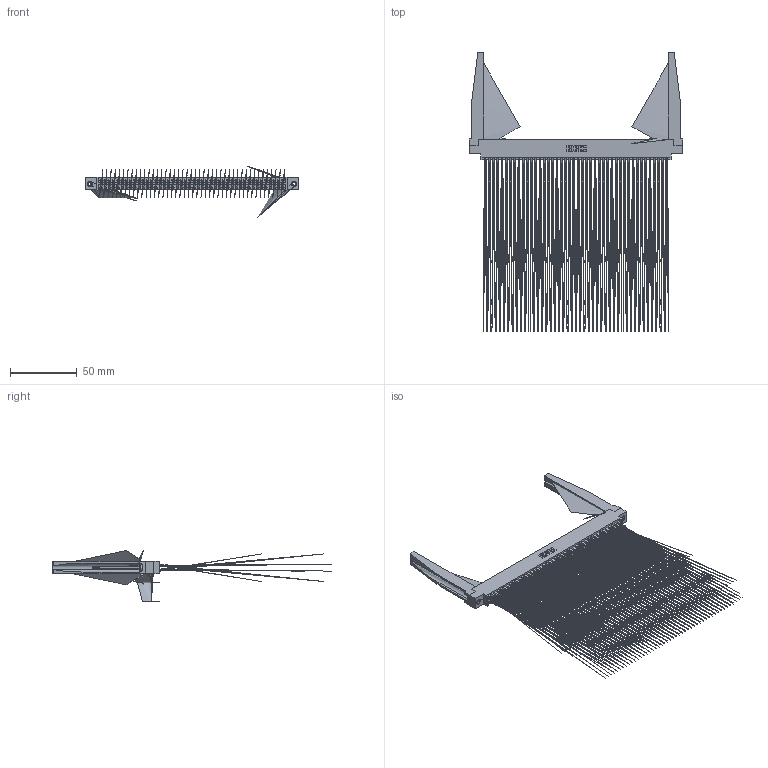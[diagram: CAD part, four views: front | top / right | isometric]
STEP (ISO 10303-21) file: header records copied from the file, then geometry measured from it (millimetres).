
FILE_DESCRIPTION (( 'STEP AP203' ), '1' );
FILE_NAME ('346-088-555-878.STEP', '2022-05-26T01:46:16', ( '' ), ( '' ), 'SwSTEP 2.0', 'SolidWorks 2020', '' );
FILE_SCHEMA (( 'CONFIG_CONTROL_DESIGN' ));
Length unit declared in the file: inch
Products named in the file (5): 345-250-001_345-250-001-102; 346 Part_0.170 Offset - 0.156 Dia-TH; 346-088-555-878; 346-220-078_345-220-078; 345-292-001_555 Tail
Assembly tree (93 placements, depth 2):
  346-088-555-878
    346 Part_0.170 Offset - 0.156 Dia-TH
    345-292-001_555 Tail  x88
    346-220-078_345-220-078  x2
    345-250-001_345-250-001-102  x2
Bounding box: 160.27 x 209.79 x 38.24 mm (x, y, z)
Volume: 24251.5 mm3; surface area: 32695.5 mm2
Topology: 93 solids, 93 shells, 5478 faces, 17093 edges, 12358 vertices
Faces by surface type: plane 3140, cylinder 2286, bspline 36, cone 12, torus 4
Entity records: 34068 total; most frequent: CARTESIAN_POINT 6591, ORIENTED_EDGE 5382, DIRECTION 4813, EDGE_CURVE 2691, VECTOR 2269, LINE 2269, VERTEX_POINT 1788, AXIS2_PLACEMENT_3D 1272
